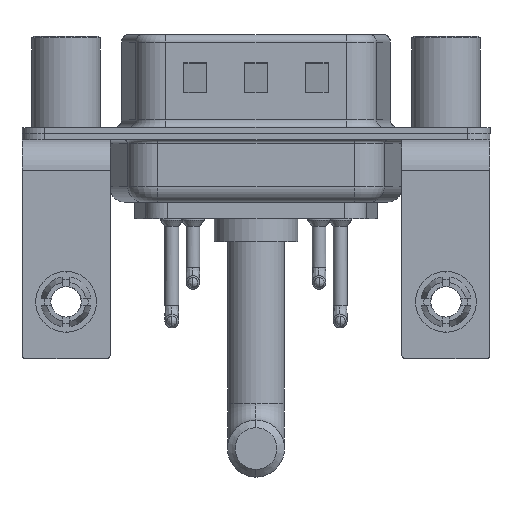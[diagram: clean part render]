
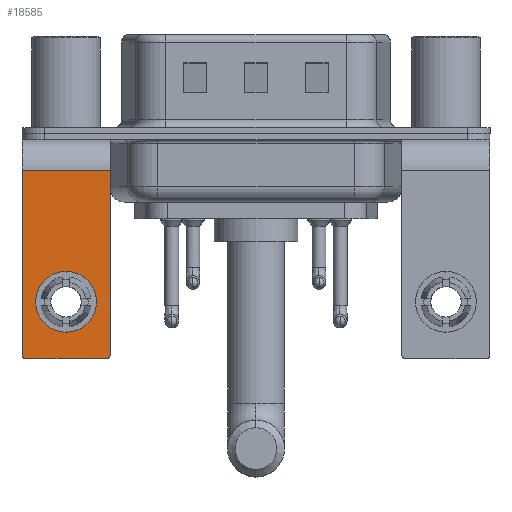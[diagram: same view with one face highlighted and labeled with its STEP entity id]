
A CAD part, front view. The second image highlights one B-rep face of the part: STEP entity #18585.
In plain terms, the highlighted planar face has unit normal (0, -1, 0).
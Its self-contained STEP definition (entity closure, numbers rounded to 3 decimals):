
#65 = EDGE_CURVE ( 'NONE', #10477, #17249, #13712, .T. ) ;
#1383 = CARTESIAN_POINT ( 'NONE',  ( -2.9, -6.25, -2.4 ) ) ;
#1405 = ORIENTED_EDGE ( 'NONE', *, *, #12899, .T. ) ;
#1960 = VERTEX_POINT ( 'NONE', #2491 ) ;
#2103 = CARTESIAN_POINT ( 'NONE',  ( -2.65, -6.25, -14.55 ) ) ;
#2208 = DIRECTION ( 'NONE',  ( 0., 0., -1. ) ) ;
#2282 = EDGE_CURVE ( 'NONE', #10477, #14593, #17898, .T. ) ;
#2491 = CARTESIAN_POINT ( 'NONE',  ( -2.9, -6.25, -14.55 ) ) ;
#2557 = DIRECTION ( 'NONE',  ( 0., 0., -1. ) ) ;
#3212 = EDGE_CURVE ( 'NONE', #15709, #13283, #13919, .T. ) ;
#3603 = DIRECTION ( 'NONE',  ( 0., -1., 0. ) ) ;
#3872 = FACE_OUTER_BOUND ( 'NONE', #3911, .T. ) ;
#3911 = EDGE_LOOP ( 'NONE', ( #21054, #1405, #11002, #19501, #7038, #17928 ) ) ;
#3950 = CARTESIAN_POINT ( 'NONE',  ( 2.9, -6.25, -2.4 ) ) ;
#3973 = LINE ( 'NONE', #11036, #8152 ) ;
#3991 = CARTESIAN_POINT ( 'NONE',  ( 2.9, -6.25, -14.8 ) ) ;
#4995 = DIRECTION ( 'NONE',  ( 0., 1., 0. ) ) ;
#5085 = CARTESIAN_POINT ( 'NONE',  ( 0., -6.25, -13.07 ) ) ;
#5103 = DIRECTION ( 'NONE',  ( 0., 0., 1. ) ) ;
#5505 = DIRECTION ( 'NONE',  ( -1., 0., 0. ) ) ;
#5808 = DIRECTION ( 'NONE',  ( 0., 0., 1. ) ) ;
#6225 = CARTESIAN_POINT ( 'NONE',  ( 2.65, -6.25, -14.55 ) ) ;
#6677 = CARTESIAN_POINT ( 'NONE',  ( 2.65, -6.25, -14.8 ) ) ;
#7038 = ORIENTED_EDGE ( 'NONE', *, *, #7953, .F. ) ;
#7462 = CARTESIAN_POINT ( 'NONE',  ( 2.9, -6.25, -14.55 ) ) ;
#7463 = EDGE_LOOP ( 'NONE', ( #13120, #22615 ) ) ;
#7467 = PLANE ( 'NONE',  #14122 ) ;
#7606 = VERTEX_POINT ( 'NONE', #10970 ) ;
#7846 = CIRCLE ( 'NONE', #22255, 0.25 ) ;
#7953 = EDGE_CURVE ( 'NONE', #7606, #17249, #21653, .T. ) ;
#8038 = CARTESIAN_POINT ( 'NONE',  ( 0., -6.25, -9.07 ) ) ;
#8152 = VECTOR ( 'NONE', #2557, 1000. ) ;
#8154 = CARTESIAN_POINT ( 'NONE',  ( 2.9, -6.25, -2.4 ) ) ;
#8185 = VECTOR ( 'NONE', #18354, 1000. ) ;
#10477 = VERTEX_POINT ( 'NONE', #6677 ) ;
#10970 = CARTESIAN_POINT ( 'NONE',  ( 2.9, -6.25, -2.4 ) ) ;
#11002 = ORIENTED_EDGE ( 'NONE', *, *, #2282, .F. ) ;
#11036 = CARTESIAN_POINT ( 'NONE',  ( -2.9, -6.25, -2.4 ) ) ;
#12801 = DIRECTION ( 'NONE',  ( 0., 0., 1. ) ) ;
#12899 = EDGE_CURVE ( 'NONE', #1960, #14593, #7846, .T. ) ;
#13120 = ORIENTED_EDGE ( 'NONE', *, *, #14501, .T. ) ;
#13283 = VERTEX_POINT ( 'NONE', #5085 ) ;
#13541 = DIRECTION ( 'NONE',  ( 0., 1., 0. ) ) ;
#13712 = CIRCLE ( 'NONE', #15934, 0.25 ) ;
#13919 = CIRCLE ( 'NONE', #14315, 2. ) ;
#13990 = DIRECTION ( 'NONE',  ( 0., 0., 1. ) ) ;
#14122 = AXIS2_PLACEMENT_3D ( 'NONE', #14536, #21578, #12801 ) ;
#14315 = AXIS2_PLACEMENT_3D ( 'NONE', #15388, #13541, #17456 ) ;
#14501 = EDGE_CURVE ( 'NONE', #13283, #15709, #18450, .T. ) ;
#14536 = CARTESIAN_POINT ( 'NONE',  ( 2.9, -6.25, -2.4 ) ) ;
#14593 = VERTEX_POINT ( 'NONE', #16440 ) ;
#15004 = LINE ( 'NONE', #8154, #8185 ) ;
#15388 = CARTESIAN_POINT ( 'NONE',  ( 0., -6.25, -11.07 ) ) ;
#15709 = VERTEX_POINT ( 'NONE', #8038 ) ;
#15934 = AXIS2_PLACEMENT_3D ( 'NONE', #6225, #22638, #13990 ) ;
#16042 = EDGE_CURVE ( 'NONE', #19050, #1960, #3973, .T. ) ;
#16440 = CARTESIAN_POINT ( 'NONE',  ( -2.65, -6.25, -14.8 ) ) ;
#16968 = EDGE_CURVE ( 'NONE', #7606, #19050, #15004, .T. ) ;
#17249 = VERTEX_POINT ( 'NONE', #7462 ) ;
#17456 = DIRECTION ( 'NONE',  ( 0., 0., 1. ) ) ;
#17898 = LINE ( 'NONE', #3991, #22704 ) ;
#17928 = ORIENTED_EDGE ( 'NONE', *, *, #16968, .T. ) ;
#18354 = DIRECTION ( 'NONE',  ( -1., 0., 0. ) ) ;
#18450 = CIRCLE ( 'NONE', #19192, 2. ) ;
#18585 = ADVANCED_FACE ( 'NONE', ( #19740, #3872 ), #7467, .F. ) ;
#19050 = VERTEX_POINT ( 'NONE', #1383 ) ;
#19192 = AXIS2_PLACEMENT_3D ( 'NONE', #20840, #4995, #5103 ) ;
#19501 = ORIENTED_EDGE ( 'NONE', *, *, #65, .T. ) ;
#19740 = FACE_BOUND ( 'NONE', #7463, .T. ) ;
#20025 = VECTOR ( 'NONE', #2208, 1000. ) ;
#20840 = CARTESIAN_POINT ( 'NONE',  ( 0., -6.25, -11.07 ) ) ;
#21054 = ORIENTED_EDGE ( 'NONE', *, *, #16042, .T. ) ;
#21578 = DIRECTION ( 'NONE',  ( 0., 1., 0. ) ) ;
#21653 = LINE ( 'NONE', #3950, #20025 ) ;
#22255 = AXIS2_PLACEMENT_3D ( 'NONE', #2103, #3603, #5808 ) ;
#22615 = ORIENTED_EDGE ( 'NONE', *, *, #3212, .T. ) ;
#22638 = DIRECTION ( 'NONE',  ( 0., -1., 0. ) ) ;
#22704 = VECTOR ( 'NONE', #5505, 1000. ) ;
